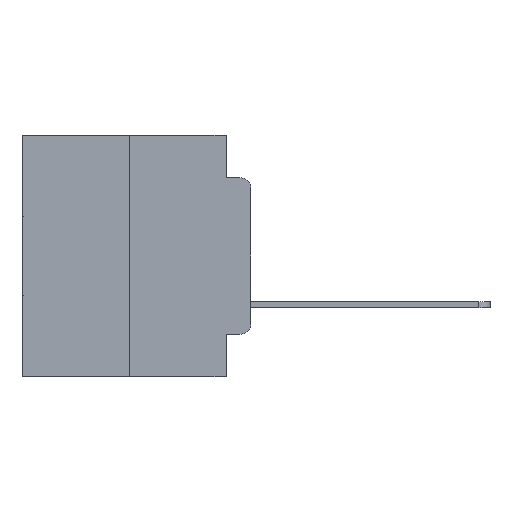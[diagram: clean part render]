
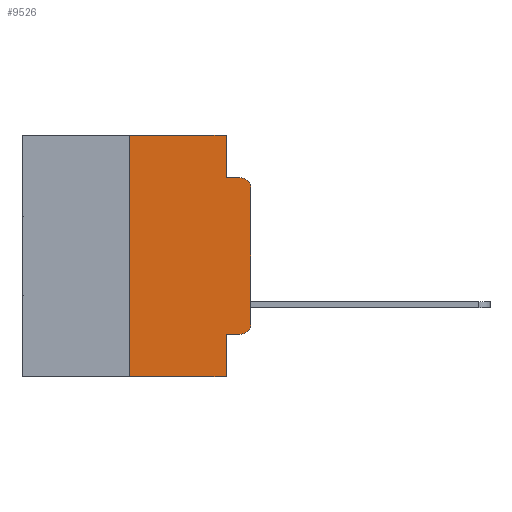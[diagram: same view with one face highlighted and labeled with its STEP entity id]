
A CAD part, left-side view. The second image highlights one B-rep face of the part: STEP entity #9526.
In plain terms, the highlighted planar face has unit normal (-1, 0, 0).
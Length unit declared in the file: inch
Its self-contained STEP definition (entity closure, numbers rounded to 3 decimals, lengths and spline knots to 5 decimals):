
#113 = DIRECTION ( 'NONE',  ( -1., 0., 0. ) ) ;
#194 = VERTEX_POINT ( 'NONE', #13137 ) ;
#309 = ORIENTED_EDGE ( 'NONE', *, *, #13501, .F. ) ;
#323 = CIRCLE ( 'NONE', #6752, 0.02 ) ;
#593 = PLANE ( 'NONE',  #17176 ) ;
#631 = ORIENTED_EDGE ( 'NONE', *, *, #2196, .F. ) ;
#941 = EDGE_LOOP ( 'NONE', ( #17227, #19222, #22225, #25561, #309, #631, #2558, #3693, #5094, #5158 ) ) ;
#959 = LINE ( 'NONE', #8718, #24561 ) ;
#1099 = DIRECTION ( 'NONE',  ( 0., -1., 0. ) ) ;
#2065 = VECTOR ( 'NONE', #1099, 39.37008 ) ;
#2196 = EDGE_CURVE ( 'NONE', #7578, #15584, #959, .T. ) ;
#2275 = CARTESIAN_POINT ( 'NONE',  ( 0., 0.02, -0.3915 ) ) ;
#2384 = CARTESIAN_POINT ( 'NONE',  ( 0., 0.25, -0.5 ) ) ;
#2558 = ORIENTED_EDGE ( 'NONE', *, *, #12646, .T. ) ;
#2980 = CARTESIAN_POINT ( 'NONE',  ( 0., 0.473, -0.5 ) ) ;
#3345 = VERTEX_POINT ( 'NONE', #18617 ) ;
#3449 = CARTESIAN_POINT ( 'NONE',  ( 0., 0.051, 0. ) ) ;
#3693 = ORIENTED_EDGE ( 'NONE', *, *, #23519, .F. ) ;
#3969 = EDGE_CURVE ( 'NONE', #25289, #9358, #21407, .T. ) ;
#4658 = DIRECTION ( 'NONE',  ( 0., 0., -1. ) ) ;
#5094 = ORIENTED_EDGE ( 'NONE', *, *, #10820, .T. ) ;
#5158 = ORIENTED_EDGE ( 'NONE', *, *, #25309, .T. ) ;
#6752 = AXIS2_PLACEMENT_3D ( 'NONE', #2275, #17953, #4658 ) ;
#7578 = VERTEX_POINT ( 'NONE', #2384 ) ;
#7619 = DIRECTION ( 'NONE',  ( 0., 0., -1. ) ) ;
#8516 = VECTOR ( 'NONE', #24916, 39.37008 ) ;
#8557 = LINE ( 'NONE', #16737, #19515 ) ;
#8718 = CARTESIAN_POINT ( 'NONE',  ( 0., 0.25, 0. ) ) ;
#9358 = VERTEX_POINT ( 'NONE', #11427 ) ;
#9526 = ADVANCED_FACE ( 'NONE', ( #9634 ), #593, .F. ) ;
#9601 = VECTOR ( 'NONE', #17276, 39.37008 ) ;
#9634 = FACE_OUTER_BOUND ( 'NONE', #941, .T. ) ;
#9642 = LINE ( 'NONE', #3449, #21193 ) ;
#10820 = EDGE_CURVE ( 'NONE', #27572, #3345, #15117, .T. ) ;
#11427 = CARTESIAN_POINT ( 'NONE',  ( 0., 0.02, -0.0885 ) ) ;
#12038 = AXIS2_PLACEMENT_3D ( 'NONE', #13772, #113, #14527 ) ;
#12646 = EDGE_CURVE ( 'NONE', #7578, #19361, #25569, .T. ) ;
#12885 = LINE ( 'NONE', #14980, #22327 ) ;
#13137 = CARTESIAN_POINT ( 'NONE',  ( 0., 0., -0.3915 ) ) ;
#13501 = EDGE_CURVE ( 'NONE', #15584, #26376, #20497, .T. ) ;
#13525 = CARTESIAN_POINT ( 'NONE',  ( 0., 0.25, 0. ) ) ;
#13772 = CARTESIAN_POINT ( 'NONE',  ( 0., 0.02, -0.1085 ) ) ;
#14527 = DIRECTION ( 'NONE',  ( 0., 0., -1. ) ) ;
#14980 = CARTESIAN_POINT ( 'NONE',  ( 0., 0.051, -0.0885 ) ) ;
#15117 = LINE ( 'NONE', #18394, #8516 ) ;
#15584 = VERTEX_POINT ( 'NONE', #13525 ) ;
#16408 = DIRECTION ( 'NONE',  ( 0., -1., 0. ) ) ;
#16737 = CARTESIAN_POINT ( 'NONE',  ( 0., 0.051, 0. ) ) ;
#16891 = CARTESIAN_POINT ( 'NONE',  ( 0., 0.473, 0. ) ) ;
#17176 = AXIS2_PLACEMENT_3D ( 'NONE', #22779, #20695, #7619 ) ;
#17227 = ORIENTED_EDGE ( 'NONE', *, *, #23689, .T. ) ;
#17276 = DIRECTION ( 'NONE',  ( 0., 0., 1. ) ) ;
#17429 = CARTESIAN_POINT ( 'NONE',  ( 0., 0.051, -0.4115 ) ) ;
#17953 = DIRECTION ( 'NONE',  ( -1., 0., 0. ) ) ;
#18394 = CARTESIAN_POINT ( 'NONE',  ( 0., 0.051, -0.4115 ) ) ;
#18604 = CARTESIAN_POINT ( 'NONE',  ( 0., 0.051, -0.0885 ) ) ;
#18617 = CARTESIAN_POINT ( 'NONE',  ( 0., 0.02, -0.4115 ) ) ;
#18862 = DIRECTION ( 'NONE',  ( 0., 0., -1. ) ) ;
#18991 = DIRECTION ( 'NONE',  ( 0., 0., -1. ) ) ;
#19222 = ORIENTED_EDGE ( 'NONE', *, *, #3969, .T. ) ;
#19361 = VERTEX_POINT ( 'NONE', #20454 ) ;
#19515 = VECTOR ( 'NONE', #18862, 39.37008 ) ;
#20247 = DIRECTION ( 'NONE',  ( 0., 0., 1. ) ) ;
#20264 = EDGE_CURVE ( 'NONE', #21277, #9358, #12885, .T. ) ;
#20454 = CARTESIAN_POINT ( 'NONE',  ( 0., 0.051, -0.5 ) ) ;
#20497 = LINE ( 'NONE', #16891, #2065 ) ;
#20695 = DIRECTION ( 'NONE',  ( 1., 0., 0. ) ) ;
#21156 = LINE ( 'NONE', #21454, #9601 ) ;
#21193 = VECTOR ( 'NONE', #18991, 39.37008 ) ;
#21277 = VERTEX_POINT ( 'NONE', #18604 ) ;
#21407 = CIRCLE ( 'NONE', #12038, 0.02 ) ;
#21454 = CARTESIAN_POINT ( 'NONE',  ( 0., 0., 0. ) ) ;
#22225 = ORIENTED_EDGE ( 'NONE', *, *, #20264, .F. ) ;
#22327 = VECTOR ( 'NONE', #27698, 39.37008 ) ;
#22779 = CARTESIAN_POINT ( 'NONE',  ( 0., 0.473, 0. ) ) ;
#23519 = EDGE_CURVE ( 'NONE', #27572, #19361, #8557, .T. ) ;
#23689 = EDGE_CURVE ( 'NONE', #194, #25289, #21156, .T. ) ;
#24225 = CARTESIAN_POINT ( 'NONE',  ( 0., 0., -0.1085 ) ) ;
#24273 = VECTOR ( 'NONE', #16408, 39.37008 ) ;
#24561 = VECTOR ( 'NONE', #20247, 39.37008 ) ;
#24916 = DIRECTION ( 'NONE',  ( 0., -1., 0. ) ) ;
#25289 = VERTEX_POINT ( 'NONE', #24225 ) ;
#25309 = EDGE_CURVE ( 'NONE', #3345, #194, #323, .T. ) ;
#25561 = ORIENTED_EDGE ( 'NONE', *, *, #26190, .F. ) ;
#25569 = LINE ( 'NONE', #2980, #24273 ) ;
#26190 = EDGE_CURVE ( 'NONE', #26376, #21277, #9642, .T. ) ;
#26376 = VERTEX_POINT ( 'NONE', #27927 ) ;
#27572 = VERTEX_POINT ( 'NONE', #17429 ) ;
#27698 = DIRECTION ( 'NONE',  ( 0., -1., 0. ) ) ;
#27927 = CARTESIAN_POINT ( 'NONE',  ( 0., 0.051, 0. ) ) ;
